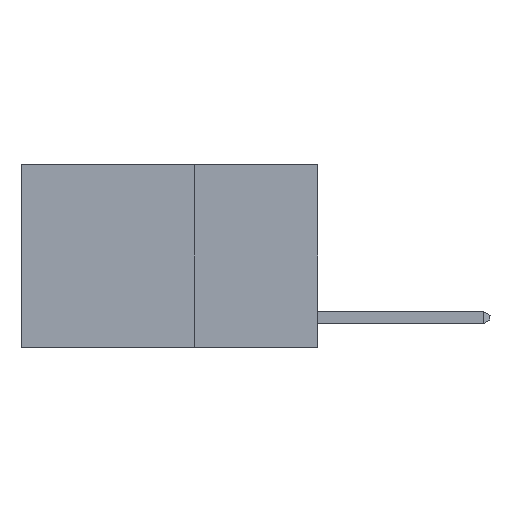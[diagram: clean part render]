
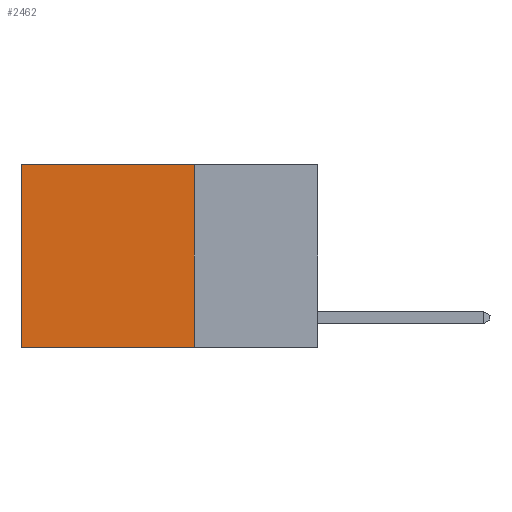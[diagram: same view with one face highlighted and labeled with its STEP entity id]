
A CAD part, left-side view. The second image highlights one B-rep face of the part: STEP entity #2462.
In plain terms, the highlighted planar face has unit normal (-1, 0, 0).
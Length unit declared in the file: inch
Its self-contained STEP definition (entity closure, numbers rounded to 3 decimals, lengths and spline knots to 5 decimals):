
#711 = LINE ( 'NONE', #5234, #9562 ) ;
#824 = EDGE_CURVE ( 'NONE', #8551, #6829, #4303, .T. ) ;
#849 = DIRECTION ( 'NONE',  ( 0., 0., -1. ) ) ;
#910 = DIRECTION ( 'NONE',  ( 0., 0., -1. ) ) ;
#2223 = DIRECTION ( 'NONE',  ( 1., 0., 0. ) ) ;
#2364 = CARTESIAN_POINT ( 'NONE',  ( 0.2625, 0.6, -0.37 ) ) ;
#2462 = ADVANCED_FACE ( 'NONE', ( #8654 ), #7775, .F. ) ;
#2614 = AXIS2_PLACEMENT_3D ( 'NONE', #4494, #2223, #910 ) ;
#3207 = DIRECTION ( 'NONE',  ( 0., 1., 0. ) ) ;
#3377 = CARTESIAN_POINT ( 'NONE',  ( 0.2625, 0.25, -0.37 ) ) ;
#3968 = EDGE_CURVE ( 'NONE', #8551, #10418, #6779, .T. ) ;
#4303 = LINE ( 'NONE', #5695, #9574 ) ;
#4494 = CARTESIAN_POINT ( 'NONE',  ( 0.2625, 0.25, 0. ) ) ;
#4905 = VECTOR ( 'NONE', #3207, 39.37008 ) ;
#5234 = CARTESIAN_POINT ( 'NONE',  ( 0.2625, 0.6, 0. ) ) ;
#5695 = CARTESIAN_POINT ( 'NONE',  ( 0.2625, 0.25, 0. ) ) ;
#5908 = VECTOR ( 'NONE', #9845, 39.37008 ) ;
#6779 = LINE ( 'NONE', #9039, #5908 ) ;
#6829 = VERTEX_POINT ( 'NONE', #9620 ) ;
#7434 = VERTEX_POINT ( 'NONE', #2364 ) ;
#7775 = PLANE ( 'NONE',  #2614 ) ;
#7970 = ORIENTED_EDGE ( 'NONE', *, *, #12501, .F. ) ;
#8551 = VERTEX_POINT ( 'NONE', #12827 ) ;
#8654 = FACE_OUTER_BOUND ( 'NONE', #12162, .T. ) ;
#9039 = CARTESIAN_POINT ( 'NONE',  ( 0.2625, 0.25, 0. ) ) ;
#9562 = VECTOR ( 'NONE', #849, 39.37008 ) ;
#9574 = VECTOR ( 'NONE', #12041, 39.37008 ) ;
#9620 = CARTESIAN_POINT ( 'NONE',  ( 0.2625, 0.6, 0. ) ) ;
#9845 = DIRECTION ( 'NONE',  ( 0., 0., -1. ) ) ;
#10418 = VERTEX_POINT ( 'NONE', #3377 ) ;
#12041 = DIRECTION ( 'NONE',  ( 0., 1., 0. ) ) ;
#12162 = EDGE_LOOP ( 'NONE', ( #13466, #7970, #13617, #12956 ) ) ;
#12256 = LINE ( 'NONE', #13280, #4905 ) ;
#12501 = EDGE_CURVE ( 'NONE', #10418, #7434, #12256, .T. ) ;
#12796 = EDGE_CURVE ( 'NONE', #6829, #7434, #711, .T. ) ;
#12827 = CARTESIAN_POINT ( 'NONE',  ( 0.2625, 0.25, 0. ) ) ;
#12956 = ORIENTED_EDGE ( 'NONE', *, *, #824, .T. ) ;
#13280 = CARTESIAN_POINT ( 'NONE',  ( 0.2625, 0.25, -0.37 ) ) ;
#13466 = ORIENTED_EDGE ( 'NONE', *, *, #12796, .T. ) ;
#13617 = ORIENTED_EDGE ( 'NONE', *, *, #3968, .F. ) ;
